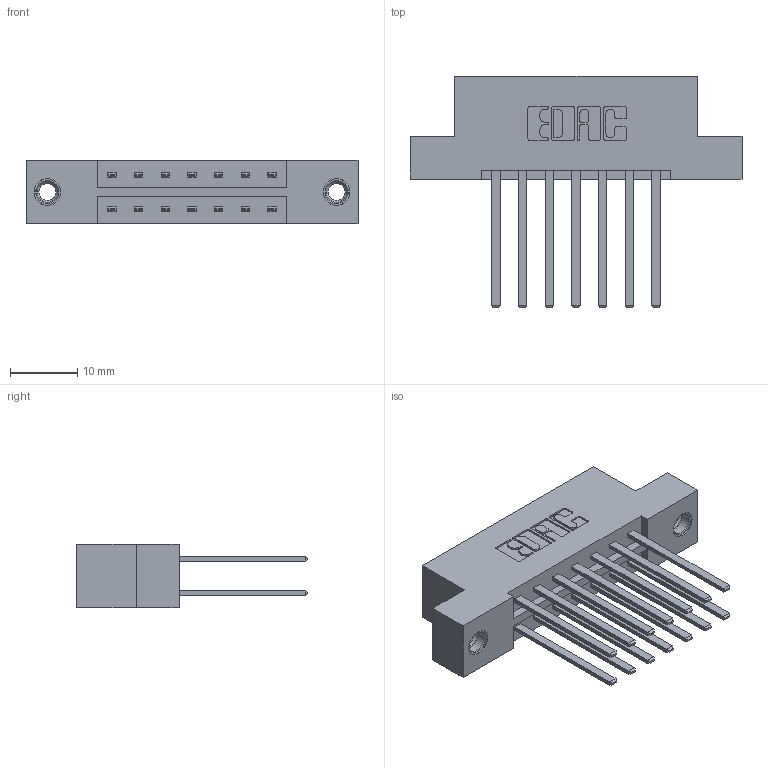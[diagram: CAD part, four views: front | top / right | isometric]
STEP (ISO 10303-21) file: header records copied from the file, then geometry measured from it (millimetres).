
FILE_DESCRIPTION (( 'STEP AP203' ), '1' );
FILE_NAME ('833-014-544-207.STEP', '2020-05-31T14:27:11', ( '' ), ( '' ), 'SwSTEP 2.0', 'SolidWorks 2020', '' );
FILE_SCHEMA (( 'CONFIG_CONTROL_DESIGN' ));
Length unit declared in the file: inch
Products named in the file (4): 833 Part_Flush - .156 Dia - TI; 345-292-001_345-293-144; 345-250-001_345-250-005-103; 833-014-544-207
Assembly tree (17 placements, depth 2):
  833-014-544-207
    833 Part_Flush - .156 Dia - TI
    345-292-001_345-293-144  x14
    345-250-001_345-250-005-103  x2
Bounding box: 49.28 x 34.3 x 9.4 mm (x, y, z)
Volume: 4886.2 mm3; surface area: 6066.7 mm2
Topology: 17 solids, 17 shells, 818 faces, 2365 edges, 1550 vertices
Faces by surface type: plane 550, cylinder 252, cone 12, torus 4
Entity records: 10032 total; most frequent: CARTESIAN_POINT 1685, ORIENTED_EDGE 1614, DIRECTION 1529, EDGE_CURVE 807, LINE 663, VECTOR 663, VERTEX_POINT 532, AXIS2_PLACEMENT_3D 433
